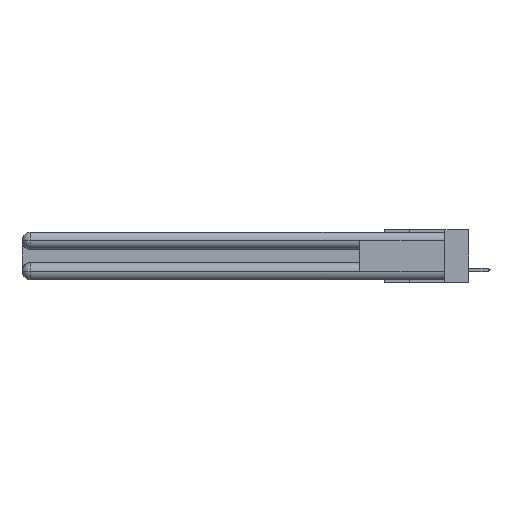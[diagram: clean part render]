
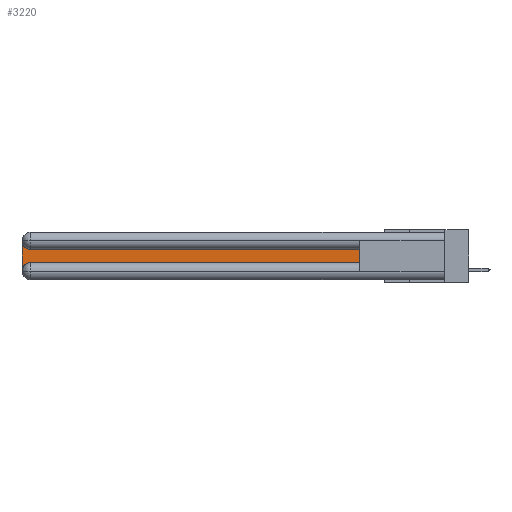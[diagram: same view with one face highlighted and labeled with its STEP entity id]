
A CAD part, left-side view. The second image highlights one B-rep face of the part: STEP entity #3220.
In plain terms, the highlighted planar face has unit normal (-1, 0, 0).
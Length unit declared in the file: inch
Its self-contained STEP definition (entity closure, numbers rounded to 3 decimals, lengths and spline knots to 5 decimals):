
#24 = CARTESIAN_POINT ( 'NONE',  ( 0.075, 3., -0.1225 ) ) ;
#219 = AXIS2_PLACEMENT_3D ( 'NONE', #24, #7531, #26312 ) ;
#752 = VECTOR ( 'NONE', #33592, 39.37008 ) ;
#3073 = CARTESIAN_POINT ( 'NONE',  ( 0.075, 2.94, -0.0625 ) ) ;
#3085 = VERTEX_POINT ( 'NONE', #17096 ) ;
#3220 = ADVANCED_FACE ( 'NONE', ( #31867 ), #13190, .F. ) ;
#3675 = DIRECTION ( 'NONE',  ( 1., 0., 0. ) ) ;
#4072 = EDGE_CURVE ( 'NONE', #8479, #19411, #24010, .T. ) ;
#5054 = LINE ( 'NONE', #5891, #11663 ) ;
#5715 = DIRECTION ( 'NONE',  ( 0., 0., -1. ) ) ;
#5891 = CARTESIAN_POINT ( 'NONE',  ( 0.075, 0.6, -0.2175 ) ) ;
#6272 = EDGE_CURVE ( 'NONE', #16236, #23701, #8996, .T. ) ;
#7531 = DIRECTION ( 'NONE',  ( 1., 0., 0. ) ) ;
#8061 = LINE ( 'NONE', #8597, #28501 ) ;
#8340 = EDGE_CURVE ( 'NONE', #3085, #8479, #8061, .T. ) ;
#8479 = VERTEX_POINT ( 'NONE', #12351 ) ;
#8597 = CARTESIAN_POINT ( 'NONE',  ( 0.075, 0.6, -0.1225 ) ) ;
#8996 = LINE ( 'NONE', #29981, #16416 ) ;
#10130 = CARTESIAN_POINT ( 'NONE',  ( 0.075, 3., -0.2175 ) ) ;
#11479 = DIRECTION ( 'NONE',  ( 0., -1., 0. ) ) ;
#11663 = VECTOR ( 'NONE', #13840, 39.37008 ) ;
#11877 = CARTESIAN_POINT ( 'NONE',  ( 0.075, 3., -0.0625 ) ) ;
#12351 = CARTESIAN_POINT ( 'NONE',  ( 0.075, 2.94, -0.1225 ) ) ;
#12744 = EDGE_LOOP ( 'NONE', ( #31486, #31707, #22255, #14049, #20273, #19524 ) ) ;
#13190 = PLANE ( 'NONE',  #219 ) ;
#13840 = DIRECTION ( 'NONE',  ( 0., 0., 1. ) ) ;
#14049 = ORIENTED_EDGE ( 'NONE', *, *, #28898, .T. ) ;
#15119 = CARTESIAN_POINT ( 'NONE',  ( 0.075, 3., -0.2775 ) ) ;
#16236 = VERTEX_POINT ( 'NONE', #29547 ) ;
#16416 = VECTOR ( 'NONE', #11479, 39.37008 ) ;
#16449 = CARTESIAN_POINT ( 'NONE',  ( 0.075, 0.6, -0.2175 ) ) ;
#17096 = CARTESIAN_POINT ( 'NONE',  ( 0.075, 0.6, -0.1225 ) ) ;
#17221 = CARTESIAN_POINT ( 'NONE',  ( 0.075, 2.94, -0.2775 ) ) ;
#19411 = VERTEX_POINT ( 'NONE', #11877 ) ;
#19524 = ORIENTED_EDGE ( 'NONE', *, *, #20532, .T. ) ;
#19826 = DIRECTION ( 'NONE',  ( 0., 0., -1. ) ) ;
#20273 = ORIENTED_EDGE ( 'NONE', *, *, #6272, .T. ) ;
#20532 = EDGE_CURVE ( 'NONE', #23701, #3085, #5054, .T. ) ;
#21395 = DIRECTION ( 'NONE',  ( 1., 0., 0. ) ) ;
#22255 = ORIENTED_EDGE ( 'NONE', *, *, #30916, .T. ) ;
#23701 = VERTEX_POINT ( 'NONE', #16449 ) ;
#24010 = CIRCLE ( 'NONE', #29448, 0.06 ) ;
#24165 = DIRECTION ( 'NONE',  ( 0., 1., 0. ) ) ;
#25123 = VERTEX_POINT ( 'NONE', #15119 ) ;
#26312 = DIRECTION ( 'NONE',  ( 0., 0., -1. ) ) ;
#28501 = VECTOR ( 'NONE', #24165, 39.37008 ) ;
#28898 = EDGE_CURVE ( 'NONE', #25123, #16236, #32876, .T. ) ;
#29448 = AXIS2_PLACEMENT_3D ( 'NONE', #3073, #21395, #5715 ) ;
#29547 = CARTESIAN_POINT ( 'NONE',  ( 0.075, 2.94, -0.2175 ) ) ;
#29981 = CARTESIAN_POINT ( 'NONE',  ( 0.075, 0.6, -0.2175 ) ) ;
#30916 = EDGE_CURVE ( 'NONE', #19411, #25123, #31515, .T. ) ;
#31486 = ORIENTED_EDGE ( 'NONE', *, *, #8340, .T. ) ;
#31515 = LINE ( 'NONE', #10130, #752 ) ;
#31707 = ORIENTED_EDGE ( 'NONE', *, *, #4072, .T. ) ;
#31867 = FACE_OUTER_BOUND ( 'NONE', #12744, .T. ) ;
#32876 = CIRCLE ( 'NONE', #33633, 0.06 ) ;
#33592 = DIRECTION ( 'NONE',  ( 0., 0., -1. ) ) ;
#33633 = AXIS2_PLACEMENT_3D ( 'NONE', #17221, #3675, #19826 ) ;
